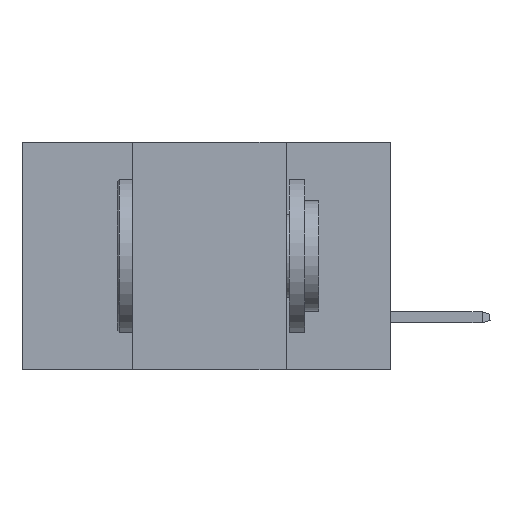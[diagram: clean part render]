
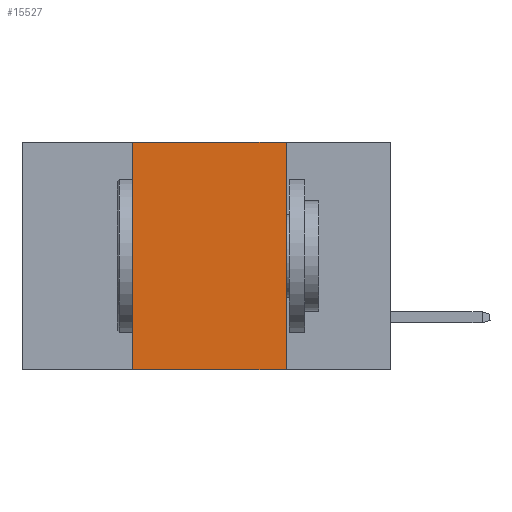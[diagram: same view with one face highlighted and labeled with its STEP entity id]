
A CAD part, left-side view. The second image highlights one B-rep face of the part: STEP entity #15527.
In plain terms, the highlighted planar face has unit normal (-1, 0, 0).
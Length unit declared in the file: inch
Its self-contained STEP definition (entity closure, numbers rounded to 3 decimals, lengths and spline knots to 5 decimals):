
#1996 = ORIENTED_EDGE ( 'NONE', *, *, #11476, .F. ) ;
#4662 = CARTESIAN_POINT ( 'NONE',  ( 0., 0.6, 0. ) ) ;
#9665 = VECTOR ( 'NONE', #21075, 39.37008 ) ;
#10125 = DIRECTION ( 'NONE',  ( 1., 0., 0. ) ) ;
#10389 = CARTESIAN_POINT ( 'NONE',  ( 0., 0.6, 0. ) ) ;
#11476 = EDGE_CURVE ( 'NONE', #14919, #15633, #12673, .T. ) ;
#11582 = ORIENTED_EDGE ( 'NONE', *, *, #21802, .T. ) ;
#11765 = EDGE_CURVE ( 'NONE', #19659, #18411, #35992, .T. ) ;
#12645 = LINE ( 'NONE', #36925, #9665 ) ;
#12673 = LINE ( 'NONE', #38121, #38500 ) ;
#14919 = VERTEX_POINT ( 'NONE', #28623 ) ;
#15264 = EDGE_LOOP ( 'NONE', ( #1996, #37329, #17871, #11582 ) ) ;
#15527 = ADVANCED_FACE ( 'NONE', ( #33244 ), #28981, .F. ) ;
#15633 = VERTEX_POINT ( 'NONE', #39985 ) ;
#16347 = DIRECTION ( 'NONE',  ( 0., 0., -1. ) ) ;
#17667 = CARTESIAN_POINT ( 'NONE',  ( 0., 0.42, -0.37 ) ) ;
#17871 = ORIENTED_EDGE ( 'NONE', *, *, #11765, .F. ) ;
#18411 = VERTEX_POINT ( 'NONE', #23520 ) ;
#19659 = VERTEX_POINT ( 'NONE', #17667 ) ;
#21075 = DIRECTION ( 'NONE',  ( 0., -1., 0. ) ) ;
#21802 = EDGE_CURVE ( 'NONE', #19659, #15633, #12645, .T. ) ;
#22384 = VECTOR ( 'NONE', #33228, 39.37008 ) ;
#23520 = CARTESIAN_POINT ( 'NONE',  ( 0., 0.42, 0. ) ) ;
#24513 = VECTOR ( 'NONE', #30448, 39.37008 ) ;
#28623 = CARTESIAN_POINT ( 'NONE',  ( 0., 0.17, 0. ) ) ;
#28879 = AXIS2_PLACEMENT_3D ( 'NONE', #10389, #10125, #16347 ) ;
#28981 = PLANE ( 'NONE',  #28879 ) ;
#30448 = DIRECTION ( 'NONE',  ( 0., 0., 1. ) ) ;
#33109 = CARTESIAN_POINT ( 'NONE',  ( 0., 0.42, 0. ) ) ;
#33228 = DIRECTION ( 'NONE',  ( 0., -1., 0. ) ) ;
#33244 = FACE_OUTER_BOUND ( 'NONE', #15264, .T. ) ;
#35992 = LINE ( 'NONE', #33109, #24513 ) ;
#36925 = CARTESIAN_POINT ( 'NONE',  ( 0., 0.6, -0.37 ) ) ;
#37329 = ORIENTED_EDGE ( 'NONE', *, *, #37451, .F. ) ;
#37339 = LINE ( 'NONE', #4662, #22384 ) ;
#37451 = EDGE_CURVE ( 'NONE', #18411, #14919, #37339, .T. ) ;
#37857 = DIRECTION ( 'NONE',  ( 0., 0., -1. ) ) ;
#38121 = CARTESIAN_POINT ( 'NONE',  ( 0., 0.17, 0. ) ) ;
#38500 = VECTOR ( 'NONE', #37857, 39.37008 ) ;
#39985 = CARTESIAN_POINT ( 'NONE',  ( 0., 0.17, -0.37 ) ) ;
